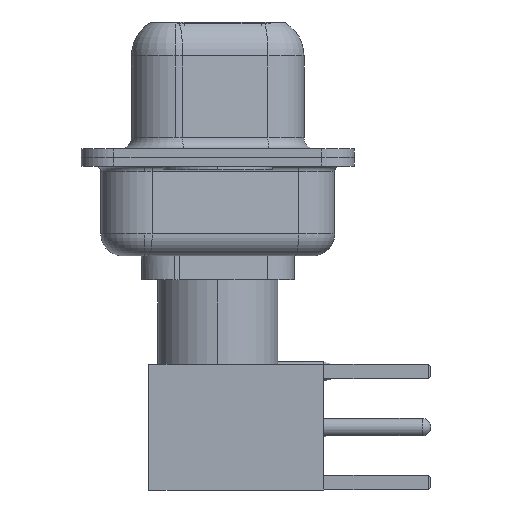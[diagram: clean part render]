
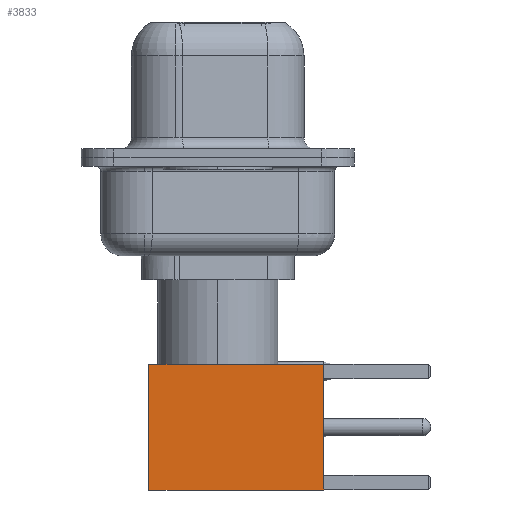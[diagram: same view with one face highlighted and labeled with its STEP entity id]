
A CAD part, left-side view. The second image highlights one B-rep face of the part: STEP entity #3833.
In plain terms, the highlighted face is planar.
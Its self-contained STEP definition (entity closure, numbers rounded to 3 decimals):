
#44 = CARTESIAN_POINT ( 'NONE',  ( -2.875, 2.875, 0. ) ) ;
#50 = ORIENTED_EDGE ( 'NONE', *, *, #15775, .F. ) ;
#849 = DIRECTION ( 'NONE',  ( -1., 0., 0. ) ) ;
#1822 = VECTOR ( 'NONE', #7062, 1000. ) ;
#1828 = VERTEX_POINT ( 'NONE', #13799 ) ;
#2799 = ORIENTED_EDGE ( 'NONE', *, *, #9096, .F. ) ;
#3162 = ORIENTED_EDGE ( 'NONE', *, *, #17641, .T. ) ;
#3833 = ADVANCED_FACE ( 'NONE', ( #10365 ), #7737, .T. ) ;
#3847 = ORIENTED_EDGE ( 'NONE', *, *, #12602, .T. ) ;
#5668 = VERTEX_POINT ( 'NONE', #7895 ) ;
#6946 = VERTEX_POINT ( 'NONE', #15643 ) ;
#7062 = DIRECTION ( 'NONE',  ( 0., 0., -1. ) ) ;
#7737 = PLANE ( 'NONE',  #17678 ) ;
#7895 = CARTESIAN_POINT ( 'NONE',  ( 2.875, 2.875, 0. ) ) ;
#8079 = EDGE_LOOP ( 'NONE', ( #3847, #3162, #50, #2799 ) ) ;
#8793 = DIRECTION ( 'NONE',  ( 0., 0., 1. ) ) ;
#9006 = VECTOR ( 'NONE', #15056, 1000. ) ;
#9010 = LINE ( 'NONE', #9286, #9506 ) ;
#9096 = EDGE_CURVE ( 'NONE', #1828, #10927, #15312, .T. ) ;
#9286 = CARTESIAN_POINT ( 'NONE',  ( 2.875, 2.875, 0. ) ) ;
#9506 = VECTOR ( 'NONE', #10769, 1000. ) ;
#10273 = CARTESIAN_POINT ( 'NONE',  ( 2.875, 2.875, 0. ) ) ;
#10365 = FACE_OUTER_BOUND ( 'NONE', #8079, .T. ) ;
#10653 = LINE ( 'NONE', #11927, #9006 ) ;
#10769 = DIRECTION ( 'NONE',  ( 0., 0., -1. ) ) ;
#10927 = VERTEX_POINT ( 'NONE', #13606 ) ;
#11927 = CARTESIAN_POINT ( 'NONE',  ( 0., 2.875, 0. ) ) ;
#12602 = EDGE_CURVE ( 'NONE', #1828, #5668, #9010, .T. ) ;
#13606 = CARTESIAN_POINT ( 'NONE',  ( -2.875, 2.875, 8. ) ) ;
#13799 = CARTESIAN_POINT ( 'NONE',  ( 2.875, 2.875, 8. ) ) ;
#15056 = DIRECTION ( 'NONE',  ( -1., 0., 0. ) ) ;
#15312 = LINE ( 'NONE', #16449, #18124 ) ;
#15553 = LINE ( 'NONE', #44, #1822 ) ;
#15643 = CARTESIAN_POINT ( 'NONE',  ( -2.875, 2.875, 0. ) ) ;
#15775 = EDGE_CURVE ( 'NONE', #10927, #6946, #15553, .T. ) ;
#15889 = DIRECTION ( 'NONE',  ( 0., 1., 0. ) ) ;
#16449 = CARTESIAN_POINT ( 'NONE',  ( 0., 2.875, 8. ) ) ;
#17641 = EDGE_CURVE ( 'NONE', #5668, #6946, #10653, .T. ) ;
#17678 = AXIS2_PLACEMENT_3D ( 'NONE', #10273, #15889, #8793 ) ;
#18124 = VECTOR ( 'NONE', #849, 1000. ) ;
